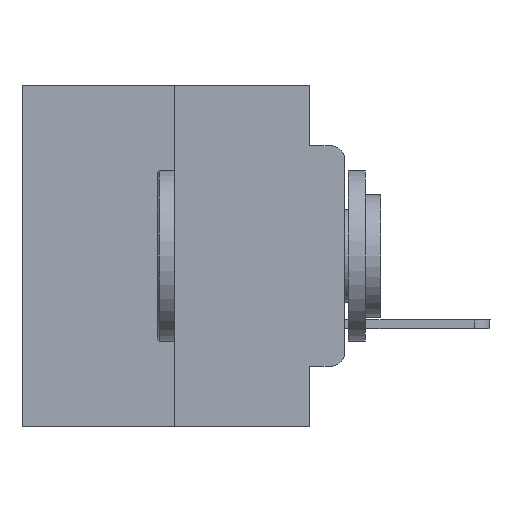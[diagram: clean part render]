
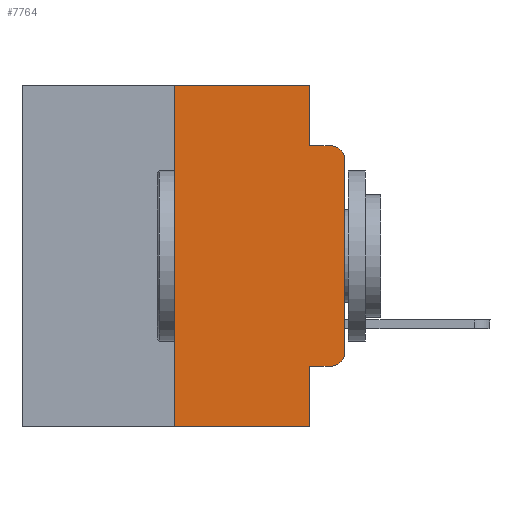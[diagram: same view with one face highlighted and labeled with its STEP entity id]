
A CAD part, left-side view. The second image highlights one B-rep face of the part: STEP entity #7764.
In plain terms, the highlighted planar face has unit normal (-1, 0, 0).
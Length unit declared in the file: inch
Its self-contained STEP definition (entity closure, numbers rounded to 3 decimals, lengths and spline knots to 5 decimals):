
#91 = EDGE_CURVE ( 'NONE', #2429, #10868, #10839, .T. ) ;
#375 = CARTESIAN_POINT ( 'NONE',  ( 0., 0.02, -0.1085 ) ) ;
#632 = LINE ( 'NONE', #23116, #3749 ) ;
#1686 = CARTESIAN_POINT ( 'NONE',  ( 0., 0.051, -0.0885 ) ) ;
#2068 = VERTEX_POINT ( 'NONE', #2359 ) ;
#2202 = VERTEX_POINT ( 'NONE', #11160 ) ;
#2359 = CARTESIAN_POINT ( 'NONE',  ( 0., 0.051, -0.4115 ) ) ;
#2429 = VERTEX_POINT ( 'NONE', #20354 ) ;
#2464 = CARTESIAN_POINT ( 'NONE',  ( 0., 0.473, -0.5 ) ) ;
#2704 = AXIS2_PLACEMENT_3D ( 'NONE', #18841, #24542, #10321 ) ;
#3127 = VERTEX_POINT ( 'NONE', #14028 ) ;
#3680 = LINE ( 'NONE', #12200, #7590 ) ;
#3749 = VECTOR ( 'NONE', #4570, 39.37008 ) ;
#3873 = VECTOR ( 'NONE', #9625, 39.37008 ) ;
#4248 = DIRECTION ( 'NONE',  ( -1., 0., 0. ) ) ;
#4570 = DIRECTION ( 'NONE',  ( 0., 0., 1. ) ) ;
#4929 = VERTEX_POINT ( 'NONE', #11152 ) ;
#5858 = LINE ( 'NONE', #22370, #3873 ) ;
#6994 = EDGE_CURVE ( 'NONE', #2068, #8125, #13112, .T. ) ;
#7035 = DIRECTION ( 'NONE',  ( 0., 0., -1. ) ) ;
#7246 = ORIENTED_EDGE ( 'NONE', *, *, #10038, .T. ) ;
#7590 = VECTOR ( 'NONE', #14108, 39.37008 ) ;
#7764 = ADVANCED_FACE ( 'NONE', ( #22915 ), #22779, .F. ) ;
#8125 = VERTEX_POINT ( 'NONE', #24099 ) ;
#8163 = DIRECTION ( 'NONE',  ( 0., -1., 0. ) ) ;
#8240 = DIRECTION ( 'NONE',  ( -1., 0., 0. ) ) ;
#8678 = VECTOR ( 'NONE', #8783, 39.37008 ) ;
#8783 = DIRECTION ( 'NONE',  ( 0., -1., 0. ) ) ;
#9625 = DIRECTION ( 'NONE',  ( 0., 0., -1. ) ) ;
#9787 = CARTESIAN_POINT ( 'NONE',  ( 0., 0., 0. ) ) ;
#10038 = EDGE_CURVE ( 'NONE', #4929, #20011, #14279, .T. ) ;
#10137 = AXIS2_PLACEMENT_3D ( 'NONE', #24946, #4248, #16839 ) ;
#10187 = LINE ( 'NONE', #2464, #24936 ) ;
#10246 = EDGE_CURVE ( 'NONE', #8125, #4929, #21849, .T. ) ;
#10321 = DIRECTION ( 'NONE',  ( 0., 0., -1. ) ) ;
#10531 = EDGE_CURVE ( 'NONE', #2202, #2429, #3680, .T. ) ;
#10759 = EDGE_LOOP ( 'NONE', ( #7246, #16088, #18269, #15579, #13202, #18320, #16059, #13642, #18075, #16877 ) ) ;
#10772 = CARTESIAN_POINT ( 'NONE',  ( 0., 0.051, -0.5 ) ) ;
#10839 = LINE ( 'NONE', #23018, #11010 ) ;
#10868 = VERTEX_POINT ( 'NONE', #13536 ) ;
#11010 = VECTOR ( 'NONE', #7035, 39.37008 ) ;
#11152 = CARTESIAN_POINT ( 'NONE',  ( 0., 0., -0.3915 ) ) ;
#11160 = CARTESIAN_POINT ( 'NONE',  ( 0., 0.25, 0. ) ) ;
#11676 = CIRCLE ( 'NONE', #14696, 0.02 ) ;
#12200 = CARTESIAN_POINT ( 'NONE',  ( 0., 0.473, 0. ) ) ;
#12571 = DIRECTION ( 'NONE',  ( 0., 0., -1. ) ) ;
#13112 = LINE ( 'NONE', #25433, #8678 ) ;
#13202 = ORIENTED_EDGE ( 'NONE', *, *, #10531, .F. ) ;
#13536 = CARTESIAN_POINT ( 'NONE',  ( 0., 0.051, -0.0885 ) ) ;
#13537 = EDGE_CURVE ( 'NONE', #3127, #2202, #632, .T. ) ;
#13642 = ORIENTED_EDGE ( 'NONE', *, *, #15966, .F. ) ;
#14028 = CARTESIAN_POINT ( 'NONE',  ( 0., 0.25, -0.5 ) ) ;
#14108 = DIRECTION ( 'NONE',  ( 0., -1., 0. ) ) ;
#14279 = LINE ( 'NONE', #9787, #14898 ) ;
#14696 = AXIS2_PLACEMENT_3D ( 'NONE', #375, #8240, #12571 ) ;
#14898 = VECTOR ( 'NONE', #16439, 39.37008 ) ;
#15515 = EDGE_CURVE ( 'NONE', #10868, #23721, #20239, .T. ) ;
#15579 = ORIENTED_EDGE ( 'NONE', *, *, #91, .F. ) ;
#15966 = EDGE_CURVE ( 'NONE', #2068, #16489, #5858, .T. ) ;
#16059 = ORIENTED_EDGE ( 'NONE', *, *, #26323, .T. ) ;
#16088 = ORIENTED_EDGE ( 'NONE', *, *, #17849, .T. ) ;
#16319 = CARTESIAN_POINT ( 'NONE',  ( 0., 0.02, -0.0885 ) ) ;
#16439 = DIRECTION ( 'NONE',  ( 0., 0., 1. ) ) ;
#16489 = VERTEX_POINT ( 'NONE', #10772 ) ;
#16839 = DIRECTION ( 'NONE',  ( 0., 0., -1. ) ) ;
#16877 = ORIENTED_EDGE ( 'NONE', *, *, #10246, .T. ) ;
#17849 = EDGE_CURVE ( 'NONE', #20011, #23721, #11676, .T. ) ;
#18075 = ORIENTED_EDGE ( 'NONE', *, *, #6994, .T. ) ;
#18269 = ORIENTED_EDGE ( 'NONE', *, *, #15515, .F. ) ;
#18320 = ORIENTED_EDGE ( 'NONE', *, *, #13537, .F. ) ;
#18329 = DIRECTION ( 'NONE',  ( 0., -1., 0. ) ) ;
#18841 = CARTESIAN_POINT ( 'NONE',  ( 0., 0.473, 0. ) ) ;
#18982 = VECTOR ( 'NONE', #18329, 39.37008 ) ;
#20011 = VERTEX_POINT ( 'NONE', #22415 ) ;
#20239 = LINE ( 'NONE', #1686, #18982 ) ;
#20354 = CARTESIAN_POINT ( 'NONE',  ( 0., 0.051, 0. ) ) ;
#21849 = CIRCLE ( 'NONE', #10137, 0.02 ) ;
#22370 = CARTESIAN_POINT ( 'NONE',  ( 0., 0.051, 0. ) ) ;
#22415 = CARTESIAN_POINT ( 'NONE',  ( 0., 0., -0.1085 ) ) ;
#22779 = PLANE ( 'NONE',  #2704 ) ;
#22915 = FACE_OUTER_BOUND ( 'NONE', #10759, .T. ) ;
#23018 = CARTESIAN_POINT ( 'NONE',  ( 0., 0.051, 0. ) ) ;
#23116 = CARTESIAN_POINT ( 'NONE',  ( 0., 0.25, 0. ) ) ;
#23721 = VERTEX_POINT ( 'NONE', #16319 ) ;
#24099 = CARTESIAN_POINT ( 'NONE',  ( 0., 0.02, -0.4115 ) ) ;
#24542 = DIRECTION ( 'NONE',  ( 1., 0., 0. ) ) ;
#24936 = VECTOR ( 'NONE', #8163, 39.37008 ) ;
#24946 = CARTESIAN_POINT ( 'NONE',  ( 0., 0.02, -0.3915 ) ) ;
#25433 = CARTESIAN_POINT ( 'NONE',  ( 0., 0.051, -0.4115 ) ) ;
#26323 = EDGE_CURVE ( 'NONE', #3127, #16489, #10187, .T. ) ;
